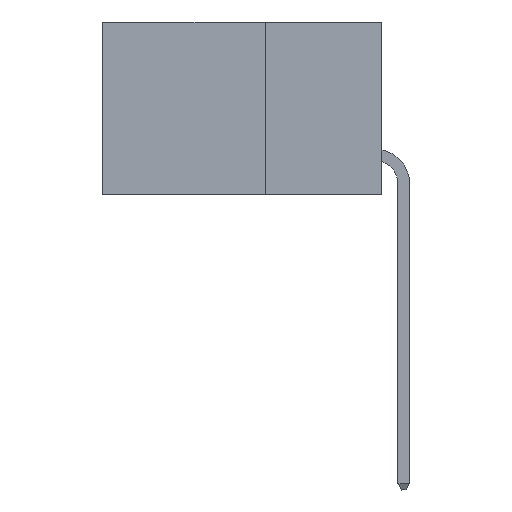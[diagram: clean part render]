
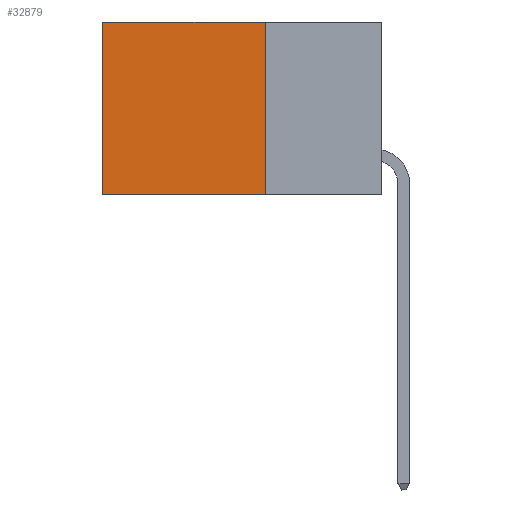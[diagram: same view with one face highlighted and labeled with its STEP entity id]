
A CAD part, left-side view. The second image highlights one B-rep face of the part: STEP entity #32879.
In plain terms, the highlighted planar face has unit normal (-1, 0, 0).
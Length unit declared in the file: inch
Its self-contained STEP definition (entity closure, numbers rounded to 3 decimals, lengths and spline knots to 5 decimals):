
#16 = LINE ( 'NONE', #16739, #8498 ) ;
#334 = CARTESIAN_POINT ( 'NONE',  ( 0.2875, 0.25, 0. ) ) ;
#1083 = VERTEX_POINT ( 'NONE', #6387 ) ;
#2786 = DIRECTION ( 'NONE',  ( 0., 0., -1. ) ) ;
#3120 = FACE_OUTER_BOUND ( 'NONE', #30498, .T. ) ;
#3211 = LINE ( 'NONE', #29441, #9416 ) ;
#3409 = VERTEX_POINT ( 'NONE', #25433 ) ;
#4132 = PLANE ( 'NONE',  #29886 ) ;
#4172 = VERTEX_POINT ( 'NONE', #4724 ) ;
#4396 = EDGE_CURVE ( 'NONE', #3409, #15591, #3211, .T. ) ;
#4662 = VECTOR ( 'NONE', #16893, 39.37008 ) ;
#4724 = CARTESIAN_POINT ( 'NONE',  ( 0.2875, 0.6, 0. ) ) ;
#6387 = CARTESIAN_POINT ( 'NONE',  ( 0.2875, 0.25, 0. ) ) ;
#7581 = EDGE_CURVE ( 'NONE', #4172, #15591, #16, .T. ) ;
#8498 = VECTOR ( 'NONE', #2786, 39.37008 ) ;
#9416 = VECTOR ( 'NONE', #44132, 39.37008 ) ;
#10295 = CARTESIAN_POINT ( 'NONE',  ( 0.2875, 0.6, -0.37 ) ) ;
#11414 = LINE ( 'NONE', #44959, #4662 ) ;
#12353 = ORIENTED_EDGE ( 'NONE', *, *, #43533, .T. ) ;
#15591 = VERTEX_POINT ( 'NONE', #10295 ) ;
#16739 = CARTESIAN_POINT ( 'NONE',  ( 0.2875, 0.6, 0. ) ) ;
#16893 = DIRECTION ( 'NONE',  ( 0., 1., 0. ) ) ;
#20270 = ORIENTED_EDGE ( 'NONE', *, *, #4396, .F. ) ;
#25433 = CARTESIAN_POINT ( 'NONE',  ( 0.2875, 0.25, -0.37 ) ) ;
#28928 = DIRECTION ( 'NONE',  ( 0., 0., -1. ) ) ;
#29244 = DIRECTION ( 'NONE',  ( 1., 0., 0. ) ) ;
#29341 = ORIENTED_EDGE ( 'NONE', *, *, #36760, .F. ) ;
#29441 = CARTESIAN_POINT ( 'NONE',  ( 0.2875, 0.25, -0.37 ) ) ;
#29886 = AXIS2_PLACEMENT_3D ( 'NONE', #334, #29244, #28928 ) ;
#30498 = EDGE_LOOP ( 'NONE', ( #40013, #20270, #29341, #12353 ) ) ;
#32879 = ADVANCED_FACE ( 'NONE', ( #3120 ), #4132, .F. ) ;
#34778 = LINE ( 'NONE', #45371, #43121 ) ;
#36760 = EDGE_CURVE ( 'NONE', #1083, #3409, #34778, .T. ) ;
#40013 = ORIENTED_EDGE ( 'NONE', *, *, #7581, .T. ) ;
#41944 = DIRECTION ( 'NONE',  ( 0., 0., -1. ) ) ;
#43121 = VECTOR ( 'NONE', #41944, 39.37008 ) ;
#43533 = EDGE_CURVE ( 'NONE', #1083, #4172, #11414, .T. ) ;
#44132 = DIRECTION ( 'NONE',  ( 0., 1., 0. ) ) ;
#44959 = CARTESIAN_POINT ( 'NONE',  ( 0.2875, 0.25, 0. ) ) ;
#45371 = CARTESIAN_POINT ( 'NONE',  ( 0.2875, 0.25, 0. ) ) ;
